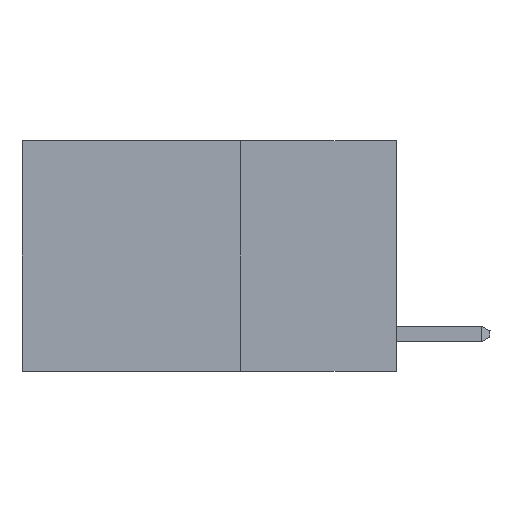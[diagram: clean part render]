
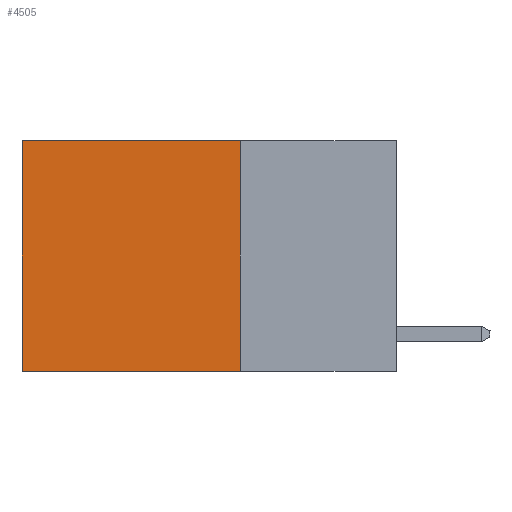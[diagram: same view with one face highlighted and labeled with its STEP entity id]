
A CAD part, left-side view. The second image highlights one B-rep face of the part: STEP entity #4505.
In plain terms, the highlighted planar face has unit normal (-1, 0, 0).
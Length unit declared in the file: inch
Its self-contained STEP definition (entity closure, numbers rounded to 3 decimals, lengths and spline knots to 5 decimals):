
#50 = FACE_OUTER_BOUND ( 'NONE', #834, .T. ) ;
#197 = CARTESIAN_POINT ( 'NONE',  ( 0.2625, 0.25, 0. ) ) ;
#720 = LINE ( 'NONE', #3749, #11992 ) ;
#834 = EDGE_LOOP ( 'NONE', ( #16677, #5195, #5102, #1512 ) ) ;
#1512 = ORIENTED_EDGE ( 'NONE', *, *, #11727, .T. ) ;
#3561 = CARTESIAN_POINT ( 'NONE',  ( 0.2625, 0.6, 0. ) ) ;
#3749 = CARTESIAN_POINT ( 'NONE',  ( 0.2625, 0.25, 0. ) ) ;
#4505 = ADVANCED_FACE ( 'NONE', ( #50 ), #9598, .F. ) ;
#4663 = DIRECTION ( 'NONE',  ( 0., 1., 0. ) ) ;
#4839 = VECTOR ( 'NONE', #10410, 39.37008 ) ;
#5102 = ORIENTED_EDGE ( 'NONE', *, *, #11066, .F. ) ;
#5137 = DIRECTION ( 'NONE',  ( 0., 1., 0. ) ) ;
#5195 = ORIENTED_EDGE ( 'NONE', *, *, #14065, .F. ) ;
#5580 = AXIS2_PLACEMENT_3D ( 'NONE', #197, #14966, #13653 ) ;
#5998 = CARTESIAN_POINT ( 'NONE',  ( 0.2625, 0.25, -0.37 ) ) ;
#6295 = VERTEX_POINT ( 'NONE', #14951 ) ;
#6828 = VECTOR ( 'NONE', #4663, 39.37008 ) ;
#7050 = CARTESIAN_POINT ( 'NONE',  ( 0.2625, 0.6, -0.37 ) ) ;
#8896 = VECTOR ( 'NONE', #14687, 39.37008 ) ;
#9549 = LINE ( 'NONE', #3561, #4839 ) ;
#9598 = PLANE ( 'NONE',  #5580 ) ;
#9817 = VERTEX_POINT ( 'NONE', #11599 ) ;
#10153 = VERTEX_POINT ( 'NONE', #16305 ) ;
#10173 = LINE ( 'NONE', #10849, #8896 ) ;
#10410 = DIRECTION ( 'NONE',  ( 0., 0., -1. ) ) ;
#10849 = CARTESIAN_POINT ( 'NONE',  ( 0.2625, 0.25, 0. ) ) ;
#11066 = EDGE_CURVE ( 'NONE', #10153, #6295, #10173, .T. ) ;
#11599 = CARTESIAN_POINT ( 'NONE',  ( 0.2625, 0.6, 0. ) ) ;
#11727 = EDGE_CURVE ( 'NONE', #10153, #9817, #720, .T. ) ;
#11992 = VECTOR ( 'NONE', #5137, 39.37008 ) ;
#13131 = LINE ( 'NONE', #5998, #6828 ) ;
#13653 = DIRECTION ( 'NONE',  ( 0., 0., -1. ) ) ;
#14065 = EDGE_CURVE ( 'NONE', #6295, #15044, #13131, .T. ) ;
#14687 = DIRECTION ( 'NONE',  ( 0., 0., -1. ) ) ;
#14802 = EDGE_CURVE ( 'NONE', #9817, #15044, #9549, .T. ) ;
#14951 = CARTESIAN_POINT ( 'NONE',  ( 0.2625, 0.25, -0.37 ) ) ;
#14966 = DIRECTION ( 'NONE',  ( 1., 0., 0. ) ) ;
#15044 = VERTEX_POINT ( 'NONE', #7050 ) ;
#16305 = CARTESIAN_POINT ( 'NONE',  ( 0.2625, 0.25, 0. ) ) ;
#16677 = ORIENTED_EDGE ( 'NONE', *, *, #14802, .T. ) ;
